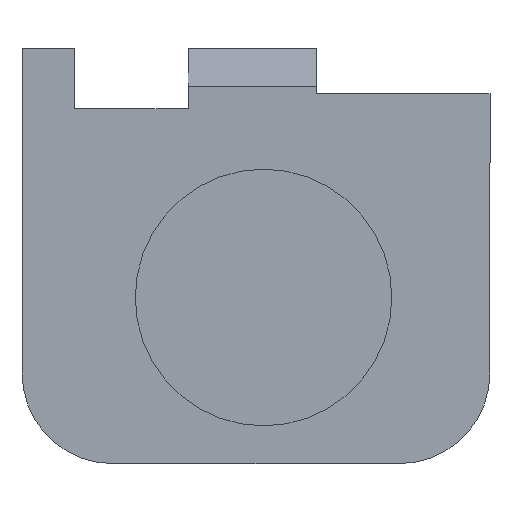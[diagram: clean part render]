
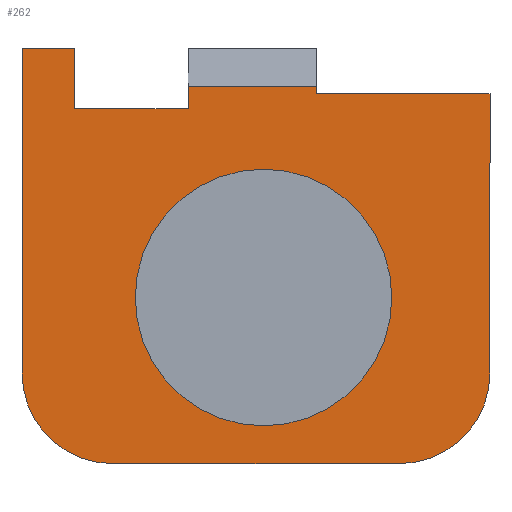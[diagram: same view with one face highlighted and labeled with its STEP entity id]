
A CAD part, front view. The second image highlights one B-rep face of the part: STEP entity #262.
In plain terms, the highlighted planar face has unit normal (0, -1, 0).
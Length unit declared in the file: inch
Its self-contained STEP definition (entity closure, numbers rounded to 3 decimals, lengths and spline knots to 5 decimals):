
#9 = LINE ( 'NONE', #643, #630 ) ;
#11 = EDGE_CURVE ( 'NONE', #628, #288, #711, .T. ) ;
#24 = VERTEX_POINT ( 'NONE', #660 ) ;
#26 = CARTESIAN_POINT ( 'NONE',  ( 0.01698, 0., 0.05431 ) ) ;
#32 = CIRCLE ( 'NONE', #670, 0.17 ) ;
#43 = VERTEX_POINT ( 'NONE', #471 ) ;
#54 = LINE ( 'NONE', #366, #718 ) ;
#58 = ORIENTED_EDGE ( 'NONE', *, *, #532, .T. ) ;
#60 = DIRECTION ( 'NONE',  ( 0., 0., -1. ) ) ;
#69 = DIRECTION ( 'NONE',  ( -1., 0., 0. ) ) ;
#70 = ORIENTED_EDGE ( 'NONE', *, *, #11, .F. ) ;
#97 = DIRECTION ( 'NONE',  ( 0., 1., 0. ) ) ;
#98 = ORIENTED_EDGE ( 'NONE', *, *, #292, .F. ) ;
#102 = VERTEX_POINT ( 'NONE', #104 ) ;
#104 = CARTESIAN_POINT ( 'NONE',  ( 0.19698, 0., -0.33569 ) ) ;
#105 = CARTESIAN_POINT ( 'NONE',  ( -0.18302, 0., -0.21569 ) ) ;
#110 = CARTESIAN_POINT ( 'NONE',  ( 0.31698, 0., -0.21569 ) ) ;
#123 = CIRCLE ( 'NONE', #617, 0.12 ) ;
#124 = ORIENTED_EDGE ( 'NONE', *, *, #234, .T. ) ;
#145 = PLANE ( 'NONE',  #271 ) ;
#157 = CARTESIAN_POINT ( 'NONE',  ( 0., 0., 0.13431 ) ) ;
#165 = DIRECTION ( 'NONE',  ( 1., 0., 0. ) ) ;
#189 = VECTOR ( 'NONE', #353, 39.37008 ) ;
#190 = DIRECTION ( 'NONE',  ( 0., 1., 0. ) ) ;
#222 = DIRECTION ( 'NONE',  ( 1., 0., 0. ) ) ;
#224 = EDGE_CURVE ( 'NONE', #636, #698, #274, .T. ) ;
#231 = EDGE_CURVE ( 'NONE', #707, #43, #9, .T. ) ;
#234 = EDGE_CURVE ( 'NONE', #730, #243, #401, .T. ) ;
#235 = VERTEX_POINT ( 'NONE', #445 ) ;
#243 = VERTEX_POINT ( 'NONE', #392 ) ;
#249 = EDGE_CURVE ( 'NONE', #243, #730, #32, .T. ) ;
#262 = ADVANCED_FACE ( 'NONE', ( #468, #716 ), #145, .F. ) ;
#265 = CARTESIAN_POINT ( 'NONE',  ( 0.01698, 0., -0.11569 ) ) ;
#271 = AXIS2_PLACEMENT_3D ( 'NONE', #536, #481, #665 ) ;
#274 = LINE ( 'NONE', #766, #340 ) ;
#275 = EDGE_CURVE ( 'NONE', #569, #43, #657, .T. ) ;
#287 = CARTESIAN_POINT ( 'NONE',  ( -0.09, 0., 0.16414 ) ) ;
#288 = VERTEX_POINT ( 'NONE', #530 ) ;
#292 = EDGE_CURVE ( 'NONE', #235, #698, #603, .T. ) ;
#297 = EDGE_CURVE ( 'NONE', #24, #102, #400, .T. ) ;
#306 = DIRECTION ( 'NONE',  ( 0., 1., 0. ) ) ;
#309 = DIRECTION ( 'NONE',  ( 0., 0., 1. ) ) ;
#322 = DIRECTION ( 'NONE',  ( 0., 0., 1. ) ) ;
#326 = VECTOR ( 'NONE', #805, 39.37008 ) ;
#340 = VECTOR ( 'NONE', #69, 39.37008 ) ;
#348 = DIRECTION ( 'NONE',  ( 0., 0., 1. ) ) ;
#353 = DIRECTION ( 'NONE',  ( -1., 0., 0. ) ) ;
#360 = CARTESIAN_POINT ( 'NONE',  ( 0.19698, 0., -0.21569 ) ) ;
#366 = CARTESIAN_POINT ( 'NONE',  ( 0.31698, 0., 0. ) ) ;
#369 = DIRECTION ( 'NONE',  ( 0., 0., 1. ) ) ;
#375 = ORIENTED_EDGE ( 'NONE', *, *, #231, .F. ) ;
#376 = AXIS2_PLACEMENT_3D ( 'NONE', #265, #190, #322 ) ;
#385 = VERTEX_POINT ( 'NONE', #110 ) ;
#387 = VECTOR ( 'NONE', #721, 39.37008 ) ;
#392 = CARTESIAN_POINT ( 'NONE',  ( 0.01698, 0., -0.28569 ) ) ;
#393 = VECTOR ( 'NONE', #222, 39.37008 ) ;
#400 = LINE ( 'NONE', #475, #731 ) ;
#401 = CIRCLE ( 'NONE', #376, 0.17 ) ;
#403 = LINE ( 'NONE', #287, #387 ) ;
#405 = CARTESIAN_POINT ( 'NONE',  ( 0.08698, 0., 0. ) ) ;
#406 = EDGE_CURVE ( 'NONE', #712, #288, #614, .T. ) ;
#418 = EDGE_CURVE ( 'NONE', #569, #628, #549, .T. ) ;
#430 = DIRECTION ( 'NONE',  ( 0., 0., 1. ) ) ;
#439 = ORIENTED_EDGE ( 'NONE', *, *, #406, .T. ) ;
#445 = CARTESIAN_POINT ( 'NONE',  ( 0.08698, 0., 0.16414 ) ) ;
#454 = CARTESIAN_POINT ( 'NONE',  ( 0.31698, 0., 0.15431 ) ) ;
#455 = AXIS2_PLACEMENT_3D ( 'NONE', #360, #306, #430 ) ;
#464 = EDGE_CURVE ( 'NONE', #707, #24, #123, .T. ) ;
#468 = FACE_BOUND ( 'NONE', #526, .T. ) ;
#471 = CARTESIAN_POINT ( 'NONE',  ( -0.30302, 0., 0.21431 ) ) ;
#475 = CARTESIAN_POINT ( 'NONE',  ( 0., 0., -0.33569 ) ) ;
#476 = ORIENTED_EDGE ( 'NONE', *, *, #517, .F. ) ;
#481 = DIRECTION ( 'NONE',  ( 0., 1., 0. ) ) ;
#495 = ORIENTED_EDGE ( 'NONE', *, *, #418, .F. ) ;
#499 = ORIENTED_EDGE ( 'NONE', *, *, #224, .T. ) ;
#505 = VECTOR ( 'NONE', #587, 39.37008 ) ;
#517 = EDGE_CURVE ( 'NONE', #385, #102, #748, .T. ) ;
#518 = VECTOR ( 'NONE', #60, 39.37008 ) ;
#526 = EDGE_LOOP ( 'NONE', ( #790, #124 ) ) ;
#530 = CARTESIAN_POINT ( 'NONE',  ( -0.08302, 0., 0.13431 ) ) ;
#532 = EDGE_CURVE ( 'NONE', #385, #636, #54, .T. ) ;
#536 = CARTESIAN_POINT ( 'NONE',  ( 0., 0., 0. ) ) ;
#549 = LINE ( 'NONE', #738, #518 ) ;
#561 = ORIENTED_EDGE ( 'NONE', *, *, #701, .F. ) ;
#564 = EDGE_LOOP ( 'NONE', ( #98, #561, #439, #70, #495, #668, #375, #599, #577, #476, #58, #499 ) ) ;
#569 = VERTEX_POINT ( 'NONE', #699 ) ;
#577 = ORIENTED_EDGE ( 'NONE', *, *, #297, .T. ) ;
#587 = DIRECTION ( 'NONE',  ( 0., 0., -1. ) ) ;
#589 = CARTESIAN_POINT ( 'NONE',  ( -0.08302, 0., 0.16414 ) ) ;
#599 = ORIENTED_EDGE ( 'NONE', *, *, #464, .T. ) ;
#603 = LINE ( 'NONE', #405, #505 ) ;
#614 = LINE ( 'NONE', #819, #326 ) ;
#617 = AXIS2_PLACEMENT_3D ( 'NONE', #105, #800, #369 ) ;
#628 = VERTEX_POINT ( 'NONE', #765 ) ;
#630 = VECTOR ( 'NONE', #757, 39.37008 ) ;
#636 = VERTEX_POINT ( 'NONE', #454 ) ;
#643 = CARTESIAN_POINT ( 'NONE',  ( -0.30302, 0., 0. ) ) ;
#657 = LINE ( 'NONE', #676, #189 ) ;
#660 = CARTESIAN_POINT ( 'NONE',  ( -0.18302, 0., -0.33569 ) ) ;
#663 = CARTESIAN_POINT ( 'NONE',  ( 0.08698, 0., 0.15431 ) ) ;
#665 = DIRECTION ( 'NONE',  ( 0., 0., 1. ) ) ;
#668 = ORIENTED_EDGE ( 'NONE', *, *, #275, .T. ) ;
#669 = CARTESIAN_POINT ( 'NONE',  ( 0.01698, 0., -0.11569 ) ) ;
#670 = AXIS2_PLACEMENT_3D ( 'NONE', #669, #97, #348 ) ;
#676 = CARTESIAN_POINT ( 'NONE',  ( 0., 0., 0.21431 ) ) ;
#698 = VERTEX_POINT ( 'NONE', #663 ) ;
#699 = CARTESIAN_POINT ( 'NONE',  ( -0.23302, 0., 0.21431 ) ) ;
#701 = EDGE_CURVE ( 'NONE', #712, #235, #403, .T. ) ;
#707 = VERTEX_POINT ( 'NONE', #725 ) ;
#711 = LINE ( 'NONE', #157, #393 ) ;
#712 = VERTEX_POINT ( 'NONE', #589 ) ;
#716 = FACE_OUTER_BOUND ( 'NONE', #564, .T. ) ;
#718 = VECTOR ( 'NONE', #309, 39.37008 ) ;
#721 = DIRECTION ( 'NONE',  ( 1., 0., 0. ) ) ;
#725 = CARTESIAN_POINT ( 'NONE',  ( -0.30302, 0., -0.21569 ) ) ;
#730 = VERTEX_POINT ( 'NONE', #26 ) ;
#731 = VECTOR ( 'NONE', #165, 39.37008 ) ;
#738 = CARTESIAN_POINT ( 'NONE',  ( -0.23302, 0., 0. ) ) ;
#748 = CIRCLE ( 'NONE', #455, 0.12 ) ;
#757 = DIRECTION ( 'NONE',  ( 0., 0., 1. ) ) ;
#765 = CARTESIAN_POINT ( 'NONE',  ( -0.23302, 0., 0.13431 ) ) ;
#766 = CARTESIAN_POINT ( 'NONE',  ( 0., 0., 0.15431 ) ) ;
#790 = ORIENTED_EDGE ( 'NONE', *, *, #249, .T. ) ;
#800 = DIRECTION ( 'NONE',  ( 0., -1., 0. ) ) ;
#805 = DIRECTION ( 'NONE',  ( 0., 0., -1. ) ) ;
#819 = CARTESIAN_POINT ( 'NONE',  ( -0.08302, 0., 0. ) ) ;
